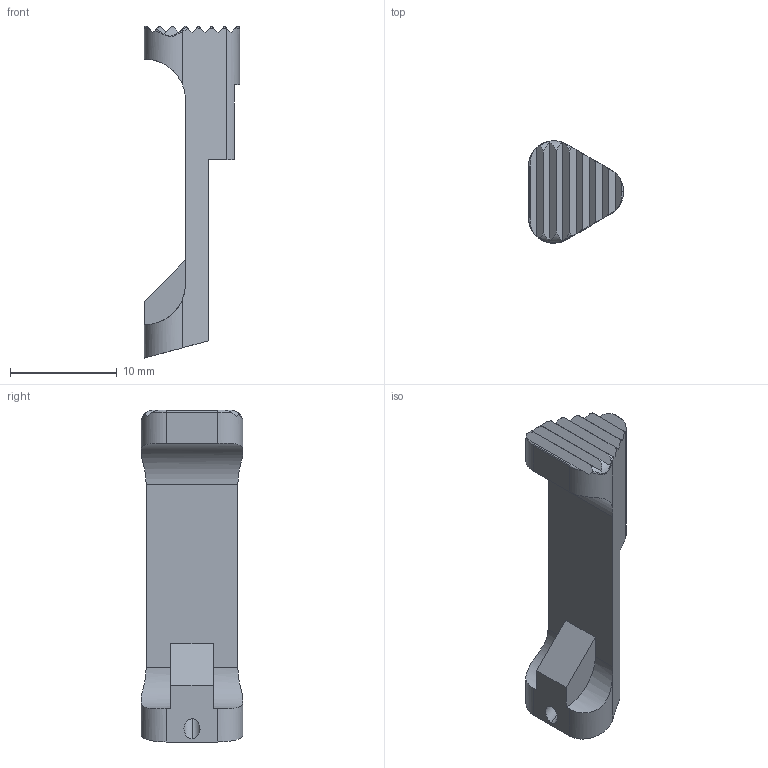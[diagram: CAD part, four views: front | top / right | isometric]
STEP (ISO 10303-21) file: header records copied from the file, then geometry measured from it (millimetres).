
FILE_DESCRIPTION (( 'STEP AP214' ), '1' );
FILE_NAME ('Magazine Catch.step', '2014-07-30T19:46:08', ( 'WarFairy' ), ( '' ), 'SwSTEP 2.0', 'SolidWorks 2013', '' );
FILE_SCHEMA (( 'AUTOMOTIVE_DESIGN' ));
Length unit declared in the file: millimetre
Products named in the file (1): Magazine Catch
Bounding box: 8.91 x 9.55 x 31.1 mm (x, y, z)
Volume: 774.5 mm3; surface area: 966.4 mm2
Topology: 1 solids, 1 shells, 78 faces, 224 edges, 147 vertices
Faces by surface type: plane 37, cylinder 29, bspline 8, torus 4
Entity records: 3012 total; most frequent: CARTESIAN_POINT 1173, ORIENTED_EDGE 448, DIRECTION 297, EDGE_CURVE 224, VERTEX_POINT 147, LINE 113, VECTOR 113, AXIS2_PLACEMENT_3D 92
